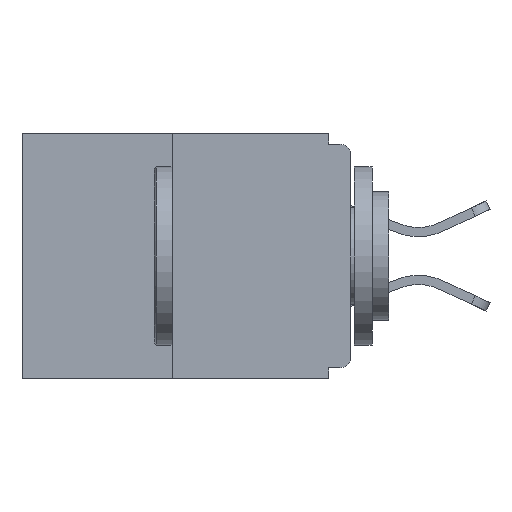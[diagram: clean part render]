
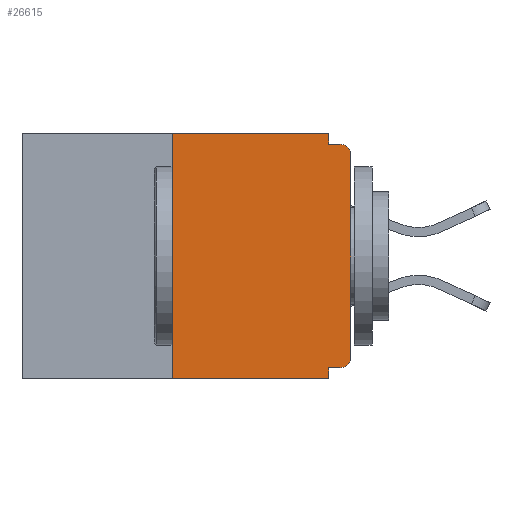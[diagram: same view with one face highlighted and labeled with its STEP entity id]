
A CAD part, left-side view. The second image highlights one B-rep face of the part: STEP entity #26615.
In plain terms, the highlighted planar face has unit normal (-1, 0, 0).
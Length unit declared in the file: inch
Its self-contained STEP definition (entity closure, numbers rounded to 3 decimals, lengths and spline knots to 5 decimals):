
#237 = ORIENTED_EDGE ( 'NONE', *, *, #6943, .F. ) ;
#1172 = ORIENTED_EDGE ( 'NONE', *, *, #23750, .F. ) ;
#1374 = PLANE ( 'NONE',  #3837 ) ;
#1817 = EDGE_CURVE ( 'NONE', #29238, #11862, #4841, .T. ) ;
#2376 = DIRECTION ( 'NONE',  ( 0., 0., 1. ) ) ;
#2659 = CARTESIAN_POINT ( 'NONE',  ( 0., 0., -0.03 ) ) ;
#2892 = CARTESIAN_POINT ( 'NONE',  ( 0., 0.015, -0.015 ) ) ;
#2992 = ORIENTED_EDGE ( 'NONE', *, *, #9574, .T. ) ;
#3588 = LINE ( 'NONE', #26961, #12400 ) ;
#3651 = ORIENTED_EDGE ( 'NONE', *, *, #17529, .F. ) ;
#3837 = AXIS2_PLACEMENT_3D ( 'NONE', #29512, #18256, #4176 ) ;
#4147 = CARTESIAN_POINT ( 'NONE',  ( 0., 0.25, 0. ) ) ;
#4176 = DIRECTION ( 'NONE',  ( 0., 0., -1. ) ) ;
#4274 = CARTESIAN_POINT ( 'NONE',  ( 0., 0.031, -0.343 ) ) ;
#4411 = CARTESIAN_POINT ( 'NONE',  ( 0., 0.031, -0.015 ) ) ;
#4691 = LINE ( 'NONE', #25798, #24486 ) ;
#4698 = CARTESIAN_POINT ( 'NONE',  ( 0., 0.031, -0.343 ) ) ;
#4841 = LINE ( 'NONE', #21749, #17353 ) ;
#5119 = VERTEX_POINT ( 'NONE', #10488 ) ;
#5238 = VERTEX_POINT ( 'NONE', #11914 ) ;
#6073 = VECTOR ( 'NONE', #18680, 39.37008 ) ;
#6631 = CARTESIAN_POINT ( 'NONE',  ( 0., 0.46, -0.343 ) ) ;
#6935 = VERTEX_POINT ( 'NONE', #27705 ) ;
#6943 = EDGE_CURVE ( 'NONE', #10335, #28616, #11203, .T. ) ;
#8329 = ORIENTED_EDGE ( 'NONE', *, *, #17117, .T. ) ;
#8868 = DIRECTION ( 'NONE',  ( -1., 0., 0. ) ) ;
#9086 = ORIENTED_EDGE ( 'NONE', *, *, #19473, .F. ) ;
#9574 = EDGE_CURVE ( 'NONE', #5119, #5238, #23730, .T. ) ;
#10057 = DIRECTION ( 'NONE',  ( 0., -1., 0. ) ) ;
#10335 = VERTEX_POINT ( 'NONE', #14607 ) ;
#10488 = CARTESIAN_POINT ( 'NONE',  ( 0., 0.015, -0.328 ) ) ;
#10611 = LINE ( 'NONE', #6631, #19815 ) ;
#10954 = DIRECTION ( 'NONE',  ( 0., 0., -1. ) ) ;
#11067 = AXIS2_PLACEMENT_3D ( 'NONE', #18466, #16225, #11247 ) ;
#11164 = VECTOR ( 'NONE', #23495, 39.37008 ) ;
#11203 = LINE ( 'NONE', #30138, #6073 ) ;
#11247 = DIRECTION ( 'NONE',  ( 0., 0., -1. ) ) ;
#11287 = VECTOR ( 'NONE', #28250, 39.37008 ) ;
#11862 = VERTEX_POINT ( 'NONE', #2892 ) ;
#11914 = CARTESIAN_POINT ( 'NONE',  ( 0., 0., -0.313 ) ) ;
#12213 = AXIS2_PLACEMENT_3D ( 'NONE', #13458, #8868, #21143 ) ;
#12382 = LINE ( 'NONE', #25772, #11287 ) ;
#12400 = VECTOR ( 'NONE', #10954, 39.37008 ) ;
#13391 = FACE_OUTER_BOUND ( 'NONE', #17038, .T. ) ;
#13458 = CARTESIAN_POINT ( 'NONE',  ( 0., 0.015, -0.03 ) ) ;
#13925 = DIRECTION ( 'NONE',  ( 0., 1., 0. ) ) ;
#14053 = EDGE_CURVE ( 'NONE', #10335, #26799, #10611, .T. ) ;
#14328 = VECTOR ( 'NONE', #13925, 39.37008 ) ;
#14607 = CARTESIAN_POINT ( 'NONE',  ( 0., 0.25, -0.343 ) ) ;
#14871 = EDGE_CURVE ( 'NONE', #28616, #6935, #12382, .T. ) ;
#16097 = DIRECTION ( 'NONE',  ( 0., -1., 0. ) ) ;
#16225 = DIRECTION ( 'NONE',  ( -1., 0., 0. ) ) ;
#16402 = ORIENTED_EDGE ( 'NONE', *, *, #1817, .F. ) ;
#16487 = CARTESIAN_POINT ( 'NONE',  ( 0., 0.031, -0.328 ) ) ;
#17038 = EDGE_LOOP ( 'NONE', ( #17920, #237, #25656, #9086, #1172, #2992, #30003, #8329, #16402, #3651 ) ) ;
#17117 = EDGE_CURVE ( 'NONE', #29422, #11862, #27474, .T. ) ;
#17353 = VECTOR ( 'NONE', #10057, 39.37008 ) ;
#17529 = EDGE_CURVE ( 'NONE', #6935, #29238, #3588, .T. ) ;
#17920 = ORIENTED_EDGE ( 'NONE', *, *, #14871, .F. ) ;
#17953 = EDGE_CURVE ( 'NONE', #5238, #29422, #4691, .T. ) ;
#18256 = DIRECTION ( 'NONE',  ( 1., 0., 0. ) ) ;
#18466 = CARTESIAN_POINT ( 'NONE',  ( 0., 0.015, -0.313 ) ) ;
#18680 = DIRECTION ( 'NONE',  ( 0., 0., 1. ) ) ;
#19473 = EDGE_CURVE ( 'NONE', #28786, #26799, #22923, .T. ) ;
#19815 = VECTOR ( 'NONE', #16097, 39.37008 ) ;
#20546 = LINE ( 'NONE', #30405, #14328 ) ;
#21143 = DIRECTION ( 'NONE',  ( 0., 0., -1. ) ) ;
#21749 = CARTESIAN_POINT ( 'NONE',  ( 0., 0., -0.015 ) ) ;
#22923 = LINE ( 'NONE', #4698, #11164 ) ;
#23495 = DIRECTION ( 'NONE',  ( 0., 0., -1. ) ) ;
#23730 = CIRCLE ( 'NONE', #11067, 0.015 ) ;
#23750 = EDGE_CURVE ( 'NONE', #5119, #28786, #20546, .T. ) ;
#24486 = VECTOR ( 'NONE', #2376, 39.37008 ) ;
#25656 = ORIENTED_EDGE ( 'NONE', *, *, #14053, .T. ) ;
#25772 = CARTESIAN_POINT ( 'NONE',  ( 0., 0.46, 0. ) ) ;
#25798 = CARTESIAN_POINT ( 'NONE',  ( 0., 0., 0. ) ) ;
#26615 = ADVANCED_FACE ( 'NONE', ( #13391 ), #1374, .F. ) ;
#26799 = VERTEX_POINT ( 'NONE', #4274 ) ;
#26961 = CARTESIAN_POINT ( 'NONE',  ( 0., 0.031, 0. ) ) ;
#27474 = CIRCLE ( 'NONE', #12213, 0.015 ) ;
#27705 = CARTESIAN_POINT ( 'NONE',  ( 0., 0.031, 0. ) ) ;
#28250 = DIRECTION ( 'NONE',  ( 0., -1., 0. ) ) ;
#28616 = VERTEX_POINT ( 'NONE', #4147 ) ;
#28786 = VERTEX_POINT ( 'NONE', #16487 ) ;
#29238 = VERTEX_POINT ( 'NONE', #4411 ) ;
#29422 = VERTEX_POINT ( 'NONE', #2659 ) ;
#29512 = CARTESIAN_POINT ( 'NONE',  ( 0., 0.46, 0. ) ) ;
#30003 = ORIENTED_EDGE ( 'NONE', *, *, #17953, .T. ) ;
#30138 = CARTESIAN_POINT ( 'NONE',  ( 0., 0.25, 0. ) ) ;
#30405 = CARTESIAN_POINT ( 'NONE',  ( 0., 0., -0.328 ) ) ;
